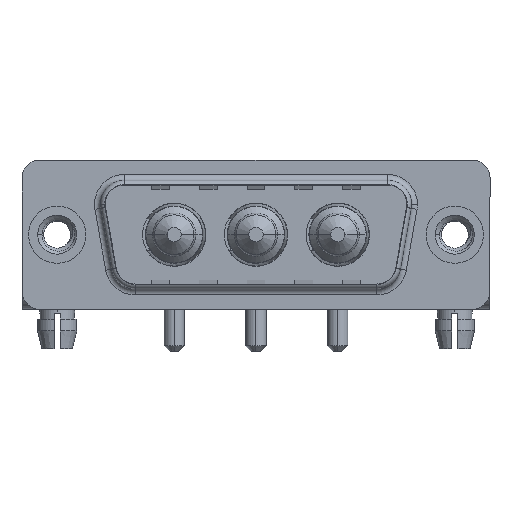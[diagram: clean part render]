
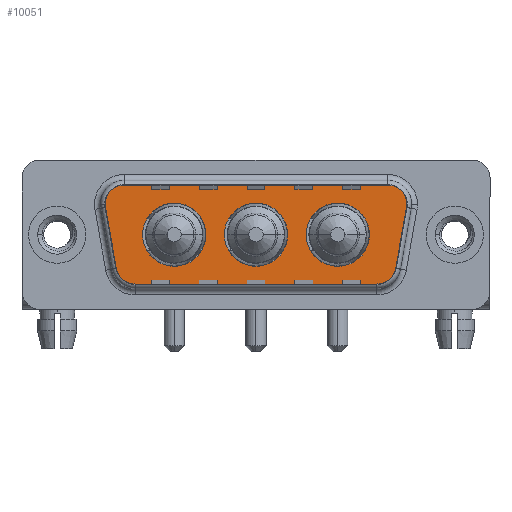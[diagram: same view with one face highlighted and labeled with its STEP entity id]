
A CAD part, top view. The second image highlights one B-rep face of the part: STEP entity #10051.
In plain terms, the highlighted planar face has unit normal (0, 0, 1).
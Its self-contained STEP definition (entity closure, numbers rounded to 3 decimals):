
#68 = DIRECTION ( 'NONE',  ( 1., 0., 0. ) ) ;
#73 = VERTEX_POINT ( 'NONE', #11616 ) ;
#129 = VERTEX_POINT ( 'NONE', #6751 ) ;
#136 = EDGE_CURVE ( 'NONE', #6670, #12524, #11476, .T. ) ;
#156 = ORIENTED_EDGE ( 'NONE', *, *, #136, .T. ) ;
#225 = EDGE_CURVE ( 'NONE', #5833, #13866, #7512, .T. ) ;
#257 = DIRECTION ( 'NONE',  ( -1., 0., 0. ) ) ;
#555 = CARTESIAN_POINT ( 'NONE',  ( 27.889, 4.9, 0. ) ) ;
#633 = CARTESIAN_POINT ( 'NONE',  ( 12.45, 0., 0. ) ) ;
#826 = DIRECTION ( 'NONE',  ( 0., 0., 1. ) ) ;
#853 = CIRCLE ( 'NONE', #2850, 2. ) ;
#885 = CARTESIAN_POINT ( 'NONE',  ( 29.859, 2.553, 0. ) ) ;
#983 = EDGE_CURVE ( 'NONE', #4592, #13072, #9295, .T. ) ;
#1113 = DIRECTION ( 'NONE',  ( 0.174, 0.985, 0. ) ) ;
#1130 = AXIS2_PLACEMENT_3D ( 'NONE', #15019, #5644, #12694 ) ;
#1324 = AXIS2_PLACEMENT_3D ( 'NONE', #1888, #4354, #9052 ) ;
#1409 = DIRECTION ( 'NONE',  ( 0., 0., 1. ) ) ;
#1443 = DIRECTION ( 'NONE',  ( -1., 0., 0. ) ) ;
#1600 = VECTOR ( 'NONE', #7535, 1000. ) ;
#1713 = CARTESIAN_POINT ( 'NONE',  ( 27.889, 2.9, 0. ) ) ;
#1799 = AXIS2_PLACEMENT_3D ( 'NONE', #10634, #6777, #68 ) ;
#1809 = CIRCLE ( 'NONE', #3295, 2.65 ) ;
#1820 = CARTESIAN_POINT ( 'NONE',  ( 28.836, -3.247, 0. ) ) ;
#1846 = DIRECTION ( 'NONE',  ( 1., 0., 0. ) ) ;
#1888 = CARTESIAN_POINT ( 'NONE',  ( 23.5, 0., 0. ) ) ;
#1928 = AXIS2_PLACEMENT_3D ( 'NONE', #6416, #13537, #4268 ) ;
#1952 = CARTESIAN_POINT ( 'NONE',  ( 6.434, -4.9, 0. ) ) ;
#2044 = VERTEX_POINT ( 'NONE', #13103 ) ;
#2291 = LINE ( 'NONE', #3851, #1600 ) ;
#2344 = VERTEX_POINT ( 'NONE', #11328 ) ;
#2652 = AXIS2_PLACEMENT_3D ( 'NONE', #12584, #11425, #1846 ) ;
#2850 = AXIS2_PLACEMENT_3D ( 'NONE', #12019, #3992, #1443 ) ;
#2921 = AXIS2_PLACEMENT_3D ( 'NONE', #10241, #9144, #10957 ) ;
#3174 = VERTEX_POINT ( 'NONE', #633 ) ;
#3204 = CARTESIAN_POINT ( 'NONE',  ( 5.411, 4.9, 0. ) ) ;
#3295 = AXIS2_PLACEMENT_3D ( 'NONE', #5602, #826, #13726 ) ;
#3824 = CARTESIAN_POINT ( 'NONE',  ( 6.434, -4.9, 0. ) ) ;
#3851 = CARTESIAN_POINT ( 'NONE',  ( 5.411, 4.9, 0. ) ) ;
#3941 = DIRECTION ( 'NONE',  ( 0., 0., 1. ) ) ;
#3949 = DIRECTION ( 'NONE',  ( 1., 0., 0. ) ) ;
#3992 = DIRECTION ( 'NONE',  ( 0., 0., 1. ) ) ;
#4150 = ORIENTED_EDGE ( 'NONE', *, *, #225, .T. ) ;
#4268 = DIRECTION ( 'NONE',  ( 1., 0., 0. ) ) ;
#4302 = CIRCLE ( 'NONE', #7503, 2. ) ;
#4354 = DIRECTION ( 'NONE',  ( 0., 0., 1. ) ) ;
#4401 = EDGE_CURVE ( 'NONE', #12524, #2044, #6975, .T. ) ;
#4544 = DIRECTION ( 'NONE',  ( 0., 0., 1. ) ) ;
#4592 = VERTEX_POINT ( 'NONE', #10273 ) ;
#4713 = ORIENTED_EDGE ( 'NONE', *, *, #983, .F. ) ;
#4728 = ORIENTED_EDGE ( 'NONE', *, *, #13250, .T. ) ;
#4852 = LINE ( 'NONE', #9634, #13898 ) ;
#5230 = EDGE_CURVE ( 'NONE', #13072, #4592, #5973, .T. ) ;
#5346 = CARTESIAN_POINT ( 'NONE',  ( 29.859, 2.553, 0. ) ) ;
#5524 = CARTESIAN_POINT ( 'NONE',  ( 9.8, 0., 0. ) ) ;
#5546 = CARTESIAN_POINT ( 'NONE',  ( 19.3, 0., 0. ) ) ;
#5602 = CARTESIAN_POINT ( 'NONE',  ( 23.5, 0., 0. ) ) ;
#5644 = DIRECTION ( 'NONE',  ( 0., 0., 1. ) ) ;
#5774 = ORIENTED_EDGE ( 'NONE', *, *, #15251, .T. ) ;
#5833 = VERTEX_POINT ( 'NONE', #1952 ) ;
#5854 = CIRCLE ( 'NONE', #1928, 2.65 ) ;
#5973 = CIRCLE ( 'NONE', #1799, 2.65 ) ;
#6275 = DIRECTION ( 'NONE',  ( 1., 0., 0. ) ) ;
#6416 = CARTESIAN_POINT ( 'NONE',  ( 9.8, 0., 0. ) ) ;
#6448 = ORIENTED_EDGE ( 'NONE', *, *, #4401, .T. ) ;
#6488 = AXIS2_PLACEMENT_3D ( 'NONE', #1713, #1409, #257 ) ;
#6670 = VERTEX_POINT ( 'NONE', #1820 ) ;
#6751 = CARTESIAN_POINT ( 'NONE',  ( 3.441, 2.553, 0. ) ) ;
#6757 = FACE_OUTER_BOUND ( 'NONE', #10717, .T. ) ;
#6777 = DIRECTION ( 'NONE',  ( 0., 0., 1. ) ) ;
#6975 = CIRCLE ( 'NONE', #6488, 2. ) ;
#7041 = ORIENTED_EDGE ( 'NONE', *, *, #10708, .T. ) ;
#7168 = CARTESIAN_POINT ( 'NONE',  ( 20.85, 0., 0. ) ) ;
#7177 = ORIENTED_EDGE ( 'NONE', *, *, #8233, .F. ) ;
#7318 = CIRCLE ( 'NONE', #9552, 2.65 ) ;
#7478 = PLANE ( 'NONE',  #2921 ) ;
#7481 = ORIENTED_EDGE ( 'NONE', *, *, #9258, .F. ) ;
#7503 = AXIS2_PLACEMENT_3D ( 'NONE', #15120, #4544, #10626 ) ;
#7510 = ORIENTED_EDGE ( 'NONE', *, *, #13921, .T. ) ;
#7512 = LINE ( 'NONE', #3824, #14762 ) ;
#7535 = DIRECTION ( 'NONE',  ( -1., 0., 0. ) ) ;
#7773 = DIRECTION ( 'NONE',  ( 0., 0., 1. ) ) ;
#7827 = CARTESIAN_POINT ( 'NONE',  ( 26.15, 0., 0. ) ) ;
#7994 = FACE_BOUND ( 'NONE', #12897, .T. ) ;
#8017 = ORIENTED_EDGE ( 'NONE', *, *, #12409, .F. ) ;
#8223 = AXIS2_PLACEMENT_3D ( 'NONE', #13343, #3941, #10950 ) ;
#8233 = EDGE_CURVE ( 'NONE', #10473, #8872, #1809, .T. ) ;
#8633 = FACE_BOUND ( 'NONE', #9539, .T. ) ;
#8872 = VERTEX_POINT ( 'NONE', #7168 ) ;
#9052 = DIRECTION ( 'NONE',  ( 1., 0., 0. ) ) ;
#9144 = DIRECTION ( 'NONE',  ( 0., 0., 1. ) ) ;
#9190 = ORIENTED_EDGE ( 'NONE', *, *, #13195, .T. ) ;
#9258 = EDGE_CURVE ( 'NONE', #8872, #10473, #11939, .T. ) ;
#9295 = CIRCLE ( 'NONE', #2652, 2.65 ) ;
#9539 = EDGE_LOOP ( 'NONE', ( #7177, #7481 ) ) ;
#9552 = AXIS2_PLACEMENT_3D ( 'NONE', #5524, #7773, #3949 ) ;
#9634 = CARTESIAN_POINT ( 'NONE',  ( 3.441, 2.553, 0. ) ) ;
#9857 = ORIENTED_EDGE ( 'NONE', *, *, #13996, .T. ) ;
#10040 = EDGE_CURVE ( 'NONE', #3174, #73, #7318, .T. ) ;
#10051 = ADVANCED_FACE ( 'NONE', ( #12199, #8633, #7994, #6757 ), #7478, .T. ) ;
#10097 = ORIENTED_EDGE ( 'NONE', *, *, #10040, .F. ) ;
#10241 = CARTESIAN_POINT ( 'NONE',  ( 26.866, -2.9, 0. ) ) ;
#10273 = CARTESIAN_POINT ( 'NONE',  ( 14., 0., 0. ) ) ;
#10473 = VERTEX_POINT ( 'NONE', #7827 ) ;
#10626 = DIRECTION ( 'NONE',  ( -1., 0., 0. ) ) ;
#10634 = CARTESIAN_POINT ( 'NONE',  ( 16.65, 0., 0. ) ) ;
#10708 = EDGE_CURVE ( 'NONE', #13866, #6670, #12482, .T. ) ;
#10717 = EDGE_LOOP ( 'NONE', ( #7041, #156, #6448, #5774, #7510, #9190, #4728, #9857, #4150 ) ) ;
#10950 = DIRECTION ( 'NONE',  ( 1., 0., 0. ) ) ;
#10957 = DIRECTION ( 'NONE',  ( 1., 0., 0. ) ) ;
#11092 = ORIENTED_EDGE ( 'NONE', *, *, #5230, .F. ) ;
#11328 = CARTESIAN_POINT ( 'NONE',  ( 4.464, -3.247, 0. ) ) ;
#11425 = DIRECTION ( 'NONE',  ( 0., 0., 1. ) ) ;
#11476 = LINE ( 'NONE', #885, #12760 ) ;
#11616 = CARTESIAN_POINT ( 'NONE',  ( 7.15, 0., 0. ) ) ;
#11663 = EDGE_LOOP ( 'NONE', ( #11092, #4713 ) ) ;
#11863 = CARTESIAN_POINT ( 'NONE',  ( 26.866, -4.9, 0. ) ) ;
#11939 = CIRCLE ( 'NONE', #1324, 2.65 ) ;
#12019 = CARTESIAN_POINT ( 'NONE',  ( 6.434, -2.9, 0. ) ) ;
#12199 = FACE_BOUND ( 'NONE', #11663, .T. ) ;
#12409 = EDGE_CURVE ( 'NONE', #73, #3174, #5854, .T. ) ;
#12468 = VERTEX_POINT ( 'NONE', #555 ) ;
#12482 = CIRCLE ( 'NONE', #1130, 2. ) ;
#12524 = VERTEX_POINT ( 'NONE', #5346 ) ;
#12584 = CARTESIAN_POINT ( 'NONE',  ( 16.65, 0., 0. ) ) ;
#12663 = CIRCLE ( 'NONE', #8223, 2. ) ;
#12694 = DIRECTION ( 'NONE',  ( 1., 0., 0. ) ) ;
#12760 = VECTOR ( 'NONE', #1113, 1000. ) ;
#12897 = EDGE_LOOP ( 'NONE', ( #10097, #8017 ) ) ;
#13072 = VERTEX_POINT ( 'NONE', #5546 ) ;
#13103 = CARTESIAN_POINT ( 'NONE',  ( 29.889, 2.9, 0. ) ) ;
#13195 = EDGE_CURVE ( 'NONE', #14575, #129, #12663, .T. ) ;
#13250 = EDGE_CURVE ( 'NONE', #129, #2344, #4852, .T. ) ;
#13343 = CARTESIAN_POINT ( 'NONE',  ( 5.411, 2.9, 0. ) ) ;
#13537 = DIRECTION ( 'NONE',  ( 0., 0., 1. ) ) ;
#13726 = DIRECTION ( 'NONE',  ( 1., 0., 0. ) ) ;
#13866 = VERTEX_POINT ( 'NONE', #11863 ) ;
#13898 = VECTOR ( 'NONE', #14279, 1000. ) ;
#13921 = EDGE_CURVE ( 'NONE', #12468, #14575, #2291, .T. ) ;
#13996 = EDGE_CURVE ( 'NONE', #2344, #5833, #853, .T. ) ;
#14279 = DIRECTION ( 'NONE',  ( 0.174, -0.985, 0. ) ) ;
#14575 = VERTEX_POINT ( 'NONE', #3204 ) ;
#14762 = VECTOR ( 'NONE', #6275, 1000. ) ;
#15019 = CARTESIAN_POINT ( 'NONE',  ( 26.866, -2.9, 0. ) ) ;
#15120 = CARTESIAN_POINT ( 'NONE',  ( 27.889, 2.9, 0. ) ) ;
#15251 = EDGE_CURVE ( 'NONE', #2044, #12468, #4302, .T. ) ;
